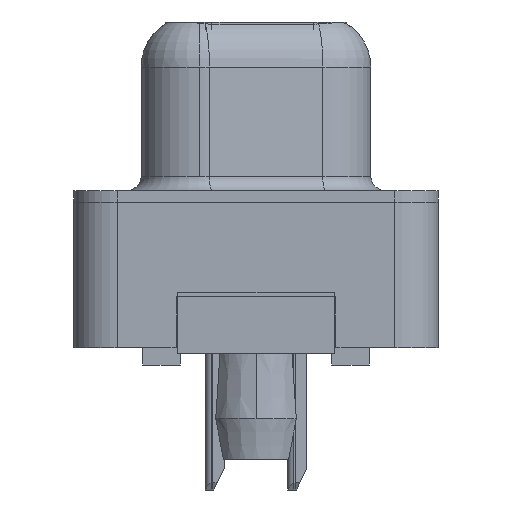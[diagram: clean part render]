
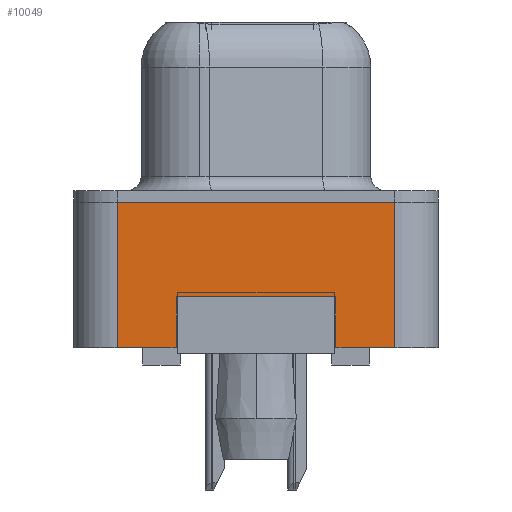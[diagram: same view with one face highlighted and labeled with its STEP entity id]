
A CAD part, left-side view. The second image highlights one B-rep face of the part: STEP entity #10049.
In plain terms, the highlighted planar face has unit normal (-1, 0, 0).
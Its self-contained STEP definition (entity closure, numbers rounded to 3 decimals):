
#88 = VERTEX_POINT ( 'NONE', #16299 ) ;
#1000 = VERTEX_POINT ( 'NONE', #8884 ) ;
#1103 = VECTOR ( 'NONE', #18426, 1000. ) ;
#1431 = EDGE_LOOP ( 'NONE', ( #11272, #22126, #13833, #17968, #15255, #23407, #15544, #12987 ) ) ;
#1997 = VECTOR ( 'NONE', #10332, 1000. ) ;
#3221 = LINE ( 'NONE', #12361, #1997 ) ;
#3403 = VECTOR ( 'NONE', #22014, 1000. ) ;
#3469 = EDGE_CURVE ( 'NONE', #10029, #1000, #13911, .T. ) ;
#4192 = DIRECTION ( 'NONE',  ( 0., 0., -1. ) ) ;
#5555 = LINE ( 'NONE', #12902, #1103 ) ;
#5898 = VERTEX_POINT ( 'NONE', #11425 ) ;
#6094 = EDGE_CURVE ( 'NONE', #15998, #5898, #3221, .T. ) ;
#7366 = LINE ( 'NONE', #14705, #3403 ) ;
#8024 = VECTOR ( 'NONE', #15938, 1000. ) ;
#8322 = DIRECTION ( 'NONE',  ( -1., 0., 0. ) ) ;
#8884 = CARTESIAN_POINT ( 'NONE',  ( -2.91, -4.775, 0. ) ) ;
#9192 = VECTOR ( 'NONE', #9363, 1000. ) ;
#9363 = DIRECTION ( 'NONE',  ( 0., 0., 1. ) ) ;
#9741 = CARTESIAN_POINT ( 'NONE',  ( -2.91, -2.75, -3.25 ) ) ;
#9852 = LINE ( 'NONE', #9741, #21838 ) ;
#10029 = VERTEX_POINT ( 'NONE', #16504 ) ;
#10049 = ADVANCED_FACE ( 'NONE', ( #11799 ), #19129, .T. ) ;
#10061 = LINE ( 'NONE', #18329, #8024 ) ;
#10332 = DIRECTION ( 'NONE',  ( 0., 0., -1. ) ) ;
#10369 = CARTESIAN_POINT ( 'NONE',  ( -2.91, 4.775, -5. ) ) ;
#10426 = CARTESIAN_POINT ( 'NONE',  ( -2.91, -4.775, 0. ) ) ;
#11272 = ORIENTED_EDGE ( 'NONE', *, *, #11839, .T. ) ;
#11347 = EDGE_CURVE ( 'NONE', #13281, #5898, #7366, .T. ) ;
#11425 = CARTESIAN_POINT ( 'NONE',  ( -2.91, 2.75, -5. ) ) ;
#11799 = FACE_OUTER_BOUND ( 'NONE', #1431, .T. ) ;
#11839 = EDGE_CURVE ( 'NONE', #21723, #88, #9852, .T. ) ;
#12102 = DIRECTION ( 'NONE',  ( 0., -1., 0. ) ) ;
#12361 = CARTESIAN_POINT ( 'NONE',  ( -2.91, 2.75, -3.25 ) ) ;
#12902 = CARTESIAN_POINT ( 'NONE',  ( -2.91, -4.775, -5. ) ) ;
#12987 = ORIENTED_EDGE ( 'NONE', *, *, #19207, .F. ) ;
#13281 = VERTEX_POINT ( 'NONE', #14716 ) ;
#13426 = LINE ( 'NONE', #18832, #9192 ) ;
#13668 = CARTESIAN_POINT ( 'NONE',  ( -2.91, 2.75, -3.25 ) ) ;
#13833 = ORIENTED_EDGE ( 'NONE', *, *, #18980, .T. ) ;
#13911 = LINE ( 'NONE', #10426, #20557 ) ;
#14705 = CARTESIAN_POINT ( 'NONE',  ( -2.91, -4.775, -5. ) ) ;
#14716 = CARTESIAN_POINT ( 'NONE',  ( -2.91, 4.775, -5. ) ) ;
#15255 = ORIENTED_EDGE ( 'NONE', *, *, #21989, .F. ) ;
#15544 = ORIENTED_EDGE ( 'NONE', *, *, #6094, .F. ) ;
#15672 = AXIS2_PLACEMENT_3D ( 'NONE', #19372, #8322, #22960 ) ;
#15938 = DIRECTION ( 'NONE',  ( 0., 1., 0. ) ) ;
#15998 = VERTEX_POINT ( 'NONE', #13668 ) ;
#16299 = CARTESIAN_POINT ( 'NONE',  ( -2.91, -2.75, -5. ) ) ;
#16504 = CARTESIAN_POINT ( 'NONE',  ( -2.91, 4.775, 0. ) ) ;
#17968 = ORIENTED_EDGE ( 'NONE', *, *, #3469, .F. ) ;
#18075 = CARTESIAN_POINT ( 'NONE',  ( -2.91, -2.75, -3.25 ) ) ;
#18329 = CARTESIAN_POINT ( 'NONE',  ( -2.91, 2.75, -3.25 ) ) ;
#18426 = DIRECTION ( 'NONE',  ( 0., -1., 0. ) ) ;
#18832 = CARTESIAN_POINT ( 'NONE',  ( -2.91, -4.775, -5. ) ) ;
#18980 = EDGE_CURVE ( 'NONE', #22417, #1000, #13426, .T. ) ;
#19129 = PLANE ( 'NONE',  #15672 ) ;
#19207 = EDGE_CURVE ( 'NONE', #21723, #15998, #10061, .T. ) ;
#19355 = CARTESIAN_POINT ( 'NONE',  ( -2.91, -4.775, -5. ) ) ;
#19372 = CARTESIAN_POINT ( 'NONE',  ( -2.91, -4.775, -5. ) ) ;
#19383 = DIRECTION ( 'NONE',  ( 0., 0., 1. ) ) ;
#19735 = EDGE_CURVE ( 'NONE', #88, #22417, #5555, .T. ) ;
#20557 = VECTOR ( 'NONE', #12102, 1000. ) ;
#20935 = LINE ( 'NONE', #10369, #22336 ) ;
#21723 = VERTEX_POINT ( 'NONE', #18075 ) ;
#21838 = VECTOR ( 'NONE', #4192, 1000. ) ;
#21989 = EDGE_CURVE ( 'NONE', #13281, #10029, #20935, .T. ) ;
#22014 = DIRECTION ( 'NONE',  ( 0., -1., 0. ) ) ;
#22126 = ORIENTED_EDGE ( 'NONE', *, *, #19735, .T. ) ;
#22336 = VECTOR ( 'NONE', #19383, 1000. ) ;
#22417 = VERTEX_POINT ( 'NONE', #19355 ) ;
#22960 = DIRECTION ( 'NONE',  ( 0., 0., 1. ) ) ;
#23407 = ORIENTED_EDGE ( 'NONE', *, *, #11347, .T. ) ;
